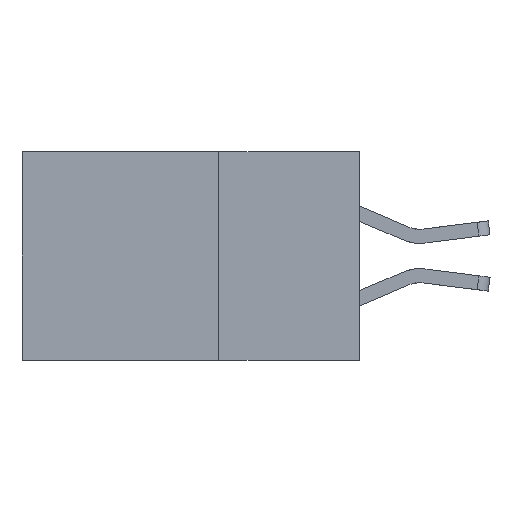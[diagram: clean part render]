
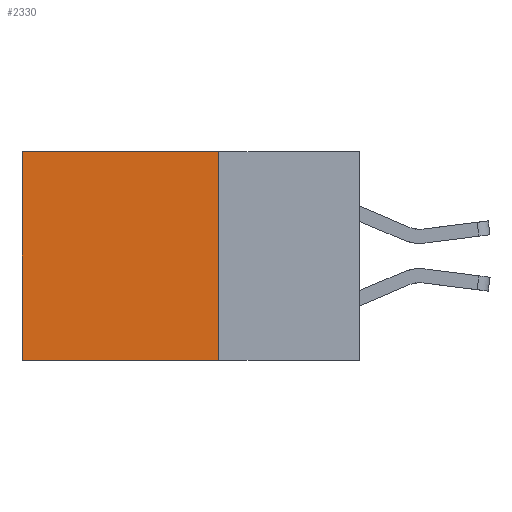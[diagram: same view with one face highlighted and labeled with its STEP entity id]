
A CAD part, left-side view. The second image highlights one B-rep face of the part: STEP entity #2330.
In plain terms, the highlighted planar face has unit normal (-1, 0, 0).
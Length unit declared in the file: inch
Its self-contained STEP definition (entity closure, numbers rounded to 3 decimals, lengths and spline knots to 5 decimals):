
#17 = VECTOR ( 'NONE', #4237, 39.37008 ) ;
#424 = VECTOR ( 'NONE', #7657, 39.37008 ) ;
#710 = CARTESIAN_POINT ( 'NONE',  ( 0.2875, 0.25, 0. ) ) ;
#1420 = DIRECTION ( 'NONE',  ( 0., 0., -1. ) ) ;
#1442 = PLANE ( 'NONE',  #4121 ) ;
#1609 = DIRECTION ( 'NONE',  ( 0., 0., -1. ) ) ;
#1746 = CARTESIAN_POINT ( 'NONE',  ( 0.2875, 0.25, -0.37 ) ) ;
#1783 = VERTEX_POINT ( 'NONE', #8125 ) ;
#2142 = CARTESIAN_POINT ( 'NONE',  ( 0.2875, 0.25, -0.37 ) ) ;
#2330 = ADVANCED_FACE ( 'NONE', ( #9151 ), #1442, .F. ) ;
#2752 = VERTEX_POINT ( 'NONE', #7097 ) ;
#2821 = LINE ( 'NONE', #5041, #17 ) ;
#3617 = ORIENTED_EDGE ( 'NONE', *, *, #5424, .F. ) ;
#3918 = VERTEX_POINT ( 'NONE', #6129 ) ;
#4121 = AXIS2_PLACEMENT_3D ( 'NONE', #7141, #9418, #7041 ) ;
#4237 = DIRECTION ( 'NONE',  ( 0., 1., 0. ) ) ;
#4958 = ORIENTED_EDGE ( 'NONE', *, *, #5007, .T. ) ;
#5007 = EDGE_CURVE ( 'NONE', #3918, #1783, #8963, .T. ) ;
#5041 = CARTESIAN_POINT ( 'NONE',  ( 0.2875, 0.25, 0. ) ) ;
#5424 = EDGE_CURVE ( 'NONE', #2752, #8854, #8679, .T. ) ;
#5610 = CARTESIAN_POINT ( 'NONE',  ( 0.2875, 0.6, 0. ) ) ;
#6129 = CARTESIAN_POINT ( 'NONE',  ( 0.2875, 0.6, 0. ) ) ;
#7041 = DIRECTION ( 'NONE',  ( 0., 0., -1. ) ) ;
#7097 = CARTESIAN_POINT ( 'NONE',  ( 0.2875, 0.25, 0. ) ) ;
#7141 = CARTESIAN_POINT ( 'NONE',  ( 0.2875, 0.25, 0. ) ) ;
#7657 = DIRECTION ( 'NONE',  ( 0., 1., 0. ) ) ;
#8125 = CARTESIAN_POINT ( 'NONE',  ( 0.2875, 0.6, -0.37 ) ) ;
#8470 = LINE ( 'NONE', #2142, #424 ) ;
#8515 = EDGE_CURVE ( 'NONE', #8854, #1783, #8470, .T. ) ;
#8620 = EDGE_LOOP ( 'NONE', ( #4958, #10026, #3617, #10193 ) ) ;
#8679 = LINE ( 'NONE', #710, #10332 ) ;
#8786 = EDGE_CURVE ( 'NONE', #2752, #3918, #2821, .T. ) ;
#8854 = VERTEX_POINT ( 'NONE', #1746 ) ;
#8963 = LINE ( 'NONE', #5610, #9602 ) ;
#9151 = FACE_OUTER_BOUND ( 'NONE', #8620, .T. ) ;
#9418 = DIRECTION ( 'NONE',  ( 1., 0., 0. ) ) ;
#9602 = VECTOR ( 'NONE', #1609, 39.37008 ) ;
#10026 = ORIENTED_EDGE ( 'NONE', *, *, #8515, .F. ) ;
#10193 = ORIENTED_EDGE ( 'NONE', *, *, #8786, .T. ) ;
#10332 = VECTOR ( 'NONE', #1420, 39.37008 ) ;
